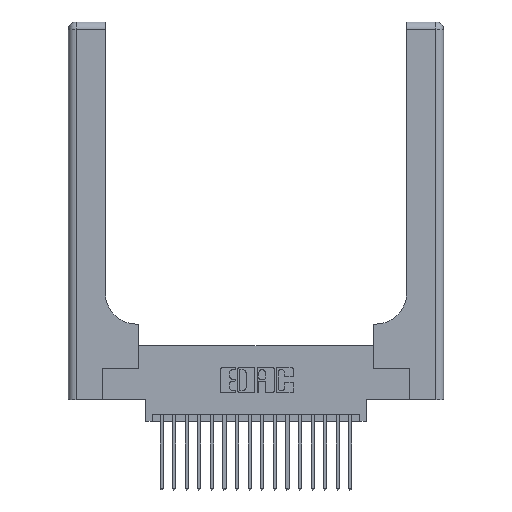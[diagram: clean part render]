
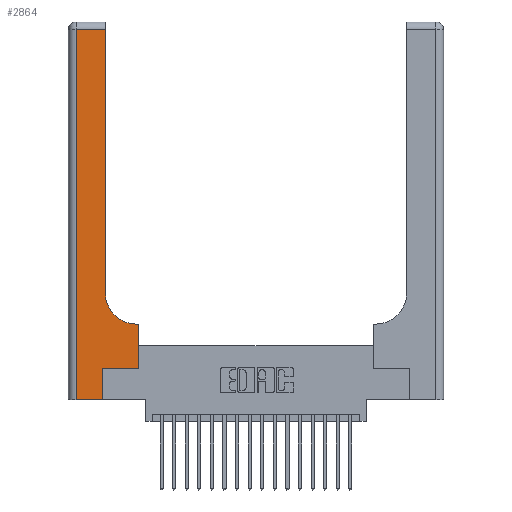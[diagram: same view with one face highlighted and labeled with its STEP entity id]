
A CAD part, top view. The second image highlights one B-rep face of the part: STEP entity #2864.
In plain terms, the highlighted planar face has unit normal (0, 0, 1).
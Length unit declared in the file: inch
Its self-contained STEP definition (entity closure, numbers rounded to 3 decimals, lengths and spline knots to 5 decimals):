
#93 = CARTESIAN_POINT ( 'NONE',  ( 0.06, 2.94, 0.37 ) ) ;
#569 = DIRECTION ( 'NONE',  ( 0., 1., 0. ) ) ;
#758 = CARTESIAN_POINT ( 'NONE',  ( 0.5415, 0.6, 0.37 ) ) ;
#883 = DIRECTION ( 'NONE',  ( 1., 0., 0. ) ) ;
#1401 = EDGE_CURVE ( 'NONE', #17074, #20795, #4165, .T. ) ;
#1470 = CARTESIAN_POINT ( 'NONE',  ( 0.5585, 0.25, 0.37 ) ) ;
#1616 = AXIS2_PLACEMENT_3D ( 'NONE', #2818, #14436, #4523 ) ;
#1843 = CARTESIAN_POINT ( 'NONE',  ( 0.2915, 0.6, 0.37 ) ) ;
#2818 = CARTESIAN_POINT ( 'NONE',  ( 0., 3., 0.37 ) ) ;
#2864 = ADVANCED_FACE ( 'NONE', ( #5158 ), #12751, .F. ) ;
#3054 = LINE ( 'NONE', #14523, #6997 ) ;
#3139 = VECTOR ( 'NONE', #569, 39.37008 ) ;
#3608 = VERTEX_POINT ( 'NONE', #19409 ) ;
#4157 = VECTOR ( 'NONE', #15179, 39.37008 ) ;
#4165 = LINE ( 'NONE', #9306, #21148 ) ;
#4359 = LINE ( 'NONE', #6606, #12628 ) ;
#4379 = VECTOR ( 'NONE', #15129, 39.37008 ) ;
#4523 = DIRECTION ( 'NONE',  ( -1., 0., 0. ) ) ;
#4909 = LINE ( 'NONE', #6783, #4379 ) ;
#5158 = FACE_OUTER_BOUND ( 'NONE', #18677, .T. ) ;
#5265 = CARTESIAN_POINT ( 'NONE',  ( 0.269, 0.25, 0.37 ) ) ;
#5428 = ORIENTED_EDGE ( 'NONE', *, *, #5840, .T. ) ;
#5705 = DIRECTION ( 'NONE',  ( 0., 0., -1. ) ) ;
#5788 = CARTESIAN_POINT ( 'NONE',  ( 0., 0., 0.37 ) ) ;
#5802 = EDGE_CURVE ( 'NONE', #17351, #20175, #7581, .T. ) ;
#5840 = EDGE_CURVE ( 'NONE', #20957, #3608, #11445, .T. ) ;
#6128 = ORIENTED_EDGE ( 'NONE', *, *, #5802, .T. ) ;
#6254 = DIRECTION ( 'NONE',  ( 0., 1., 0. ) ) ;
#6606 = CARTESIAN_POINT ( 'NONE',  ( 0.2915, 3., 0.37 ) ) ;
#6679 = EDGE_CURVE ( 'NONE', #20175, #20957, #17384, .T. ) ;
#6783 = CARTESIAN_POINT ( 'NONE',  ( 0.06, 3., 0.37 ) ) ;
#6997 = VECTOR ( 'NONE', #9596, 39.37008 ) ;
#7453 = DIRECTION ( 'NONE',  ( 1., 0., 0. ) ) ;
#7581 = LINE ( 'NONE', #20364, #3139 ) ;
#7740 = EDGE_CURVE ( 'NONE', #21277, #11218, #3054, .T. ) ;
#7847 = ORIENTED_EDGE ( 'NONE', *, *, #10777, .T. ) ;
#7898 = EDGE_CURVE ( 'NONE', #11218, #12363, #4909, .T. ) ;
#8252 = CARTESIAN_POINT ( 'NONE',  ( 0.5585, 0.6, 0.37 ) ) ;
#8265 = DIRECTION ( 'NONE',  ( 0., 1., 0. ) ) ;
#8434 = EDGE_CURVE ( 'NONE', #3608, #21277, #4359, .T. ) ;
#9294 = AXIS2_PLACEMENT_3D ( 'NONE', #15640, #5705, #17284 ) ;
#9306 = CARTESIAN_POINT ( 'NONE',  ( 0.269, 0., 0.37 ) ) ;
#9596 = DIRECTION ( 'NONE',  ( -1., 0., 0. ) ) ;
#9999 = VECTOR ( 'NONE', #7453, 39.37008 ) ;
#10182 = EDGE_CURVE ( 'NONE', #20795, #17351, #13094, .T. ) ;
#10294 = ORIENTED_EDGE ( 'NONE', *, *, #8434, .T. ) ;
#10503 = LINE ( 'NONE', #5788, #9999 ) ;
#10777 = EDGE_CURVE ( 'NONE', #12363, #17074, #10503, .T. ) ;
#11218 = VERTEX_POINT ( 'NONE', #93 ) ;
#11445 = CIRCLE ( 'NONE', #9294, 0.25 ) ;
#12363 = VERTEX_POINT ( 'NONE', #16036 ) ;
#12628 = VECTOR ( 'NONE', #8265, 39.37008 ) ;
#12751 = PLANE ( 'NONE',  #1616 ) ;
#13094 = LINE ( 'NONE', #15814, #20792 ) ;
#13763 = ORIENTED_EDGE ( 'NONE', *, *, #7898, .T. ) ;
#14436 = DIRECTION ( 'NONE',  ( 0., 0., -1. ) ) ;
#14523 = CARTESIAN_POINT ( 'NONE',  ( 0., 2.94, 0.37 ) ) ;
#15129 = DIRECTION ( 'NONE',  ( 0., -1., 0. ) ) ;
#15179 = DIRECTION ( 'NONE',  ( -1., 0., 0. ) ) ;
#15640 = CARTESIAN_POINT ( 'NONE',  ( 0.5415, 0.85, 0.37 ) ) ;
#15814 = CARTESIAN_POINT ( 'NONE',  ( 0.269, 0.25, 0.37 ) ) ;
#16036 = CARTESIAN_POINT ( 'NONE',  ( 0.06, 0., 0.37 ) ) ;
#16380 = ORIENTED_EDGE ( 'NONE', *, *, #6679, .T. ) ;
#16488 = ORIENTED_EDGE ( 'NONE', *, *, #10182, .T. ) ;
#17074 = VERTEX_POINT ( 'NONE', #18171 ) ;
#17284 = DIRECTION ( 'NONE',  ( 1., 0., 0. ) ) ;
#17351 = VERTEX_POINT ( 'NONE', #1470 ) ;
#17384 = LINE ( 'NONE', #1843, #4157 ) ;
#18043 = ORIENTED_EDGE ( 'NONE', *, *, #7740, .T. ) ;
#18171 = CARTESIAN_POINT ( 'NONE',  ( 0.269, 0., 0.37 ) ) ;
#18677 = EDGE_LOOP ( 'NONE', ( #10294, #18043, #13763, #7847, #20893, #16488, #6128, #16380, #5428 ) ) ;
#19409 = CARTESIAN_POINT ( 'NONE',  ( 0.2915, 0.85, 0.37 ) ) ;
#19757 = CARTESIAN_POINT ( 'NONE',  ( 0.2915, 2.94, 0.37 ) ) ;
#20175 = VERTEX_POINT ( 'NONE', #8252 ) ;
#20364 = CARTESIAN_POINT ( 'NONE',  ( 0.5585, 0.25, 0.37 ) ) ;
#20792 = VECTOR ( 'NONE', #883, 39.37008 ) ;
#20795 = VERTEX_POINT ( 'NONE', #5265 ) ;
#20893 = ORIENTED_EDGE ( 'NONE', *, *, #1401, .T. ) ;
#20957 = VERTEX_POINT ( 'NONE', #758 ) ;
#21148 = VECTOR ( 'NONE', #6254, 39.37008 ) ;
#21277 = VERTEX_POINT ( 'NONE', #19757 ) ;
